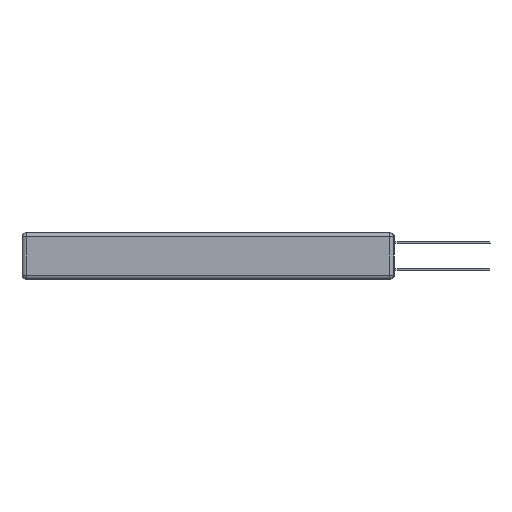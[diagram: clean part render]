
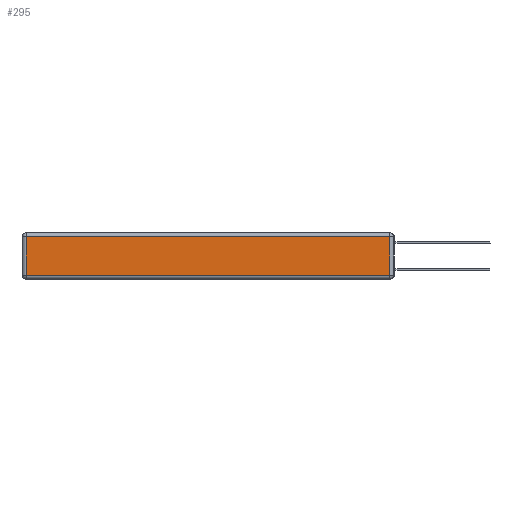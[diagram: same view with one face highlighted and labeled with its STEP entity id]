
A CAD part, left-side view. The second image highlights one B-rep face of the part: STEP entity #295.
In plain terms, the highlighted planar face has unit normal (-1, 0, 0).
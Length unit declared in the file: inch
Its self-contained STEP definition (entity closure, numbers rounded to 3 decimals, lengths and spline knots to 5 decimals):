
#295 = ADVANCED_FACE ( 'NONE', ( #11192 ), #3622, .T. ) ;
#311 = VERTEX_POINT ( 'NONE', #17973 ) ;
#395 = CARTESIAN_POINT ( 'NONE',  ( 0., 0.03, -0.343 ) ) ;
#1920 = VERTEX_POINT ( 'NONE', #8282 ) ;
#2831 = VECTOR ( 'NONE', #11084, 39.37008 ) ;
#3622 = PLANE ( 'NONE',  #17359 ) ;
#3855 = VECTOR ( 'NONE', #4926, 39.37008 ) ;
#4410 = VERTEX_POINT ( 'NONE', #5360 ) ;
#4788 = CARTESIAN_POINT ( 'NONE',  ( 0., 0., -0.313 ) ) ;
#4836 = CARTESIAN_POINT ( 'NONE',  ( 0., 2.75, -0.03 ) ) ;
#4926 = DIRECTION ( 'NONE',  ( 0., 0., 1. ) ) ;
#5360 = CARTESIAN_POINT ( 'NONE',  ( 0., 2.72, -0.313 ) ) ;
#7229 = CARTESIAN_POINT ( 'NONE',  ( 0., 2.72, -0.03 ) ) ;
#7835 = CARTESIAN_POINT ( 'NONE',  ( 0., 2.72, -0.343 ) ) ;
#8282 = CARTESIAN_POINT ( 'NONE',  ( 0., 0.03, -0.313 ) ) ;
#8503 = DIRECTION ( 'NONE',  ( 0., 0., 1. ) ) ;
#8629 = EDGE_CURVE ( 'NONE', #4410, #1920, #18744, .T. ) ;
#10493 = ORIENTED_EDGE ( 'NONE', *, *, #8629, .T. ) ;
#11084 = DIRECTION ( 'NONE',  ( 0., 1., 0. ) ) ;
#11160 = LINE ( 'NONE', #395, #3855 ) ;
#11192 = FACE_OUTER_BOUND ( 'NONE', #18232, .T. ) ;
#11782 = VERTEX_POINT ( 'NONE', #7229 ) ;
#12375 = VECTOR ( 'NONE', #14061, 39.37008 ) ;
#12714 = ORIENTED_EDGE ( 'NONE', *, *, #19659, .T. ) ;
#12901 = LINE ( 'NONE', #4836, #2831 ) ;
#13052 = ORIENTED_EDGE ( 'NONE', *, *, #17495, .T. ) ;
#14061 = DIRECTION ( 'NONE',  ( 0., 0., -1. ) ) ;
#14818 = CARTESIAN_POINT ( 'NONE',  ( 0., 0., -0.343 ) ) ;
#14919 = DIRECTION ( 'NONE',  ( -1., 0., 0. ) ) ;
#15565 = LINE ( 'NONE', #7835, #12375 ) ;
#15612 = VECTOR ( 'NONE', #17217, 39.37008 ) ;
#15764 = ORIENTED_EDGE ( 'NONE', *, *, #15854, .T. ) ;
#15854 = EDGE_CURVE ( 'NONE', #311, #11782, #12901, .T. ) ;
#17217 = DIRECTION ( 'NONE',  ( 0., -1., 0. ) ) ;
#17359 = AXIS2_PLACEMENT_3D ( 'NONE', #14818, #14919, #8503 ) ;
#17495 = EDGE_CURVE ( 'NONE', #1920, #311, #11160, .T. ) ;
#17973 = CARTESIAN_POINT ( 'NONE',  ( 0., 0.03, -0.03 ) ) ;
#18232 = EDGE_LOOP ( 'NONE', ( #10493, #13052, #15764, #12714 ) ) ;
#18744 = LINE ( 'NONE', #4788, #15612 ) ;
#19659 = EDGE_CURVE ( 'NONE', #11782, #4410, #15565, .T. ) ;
